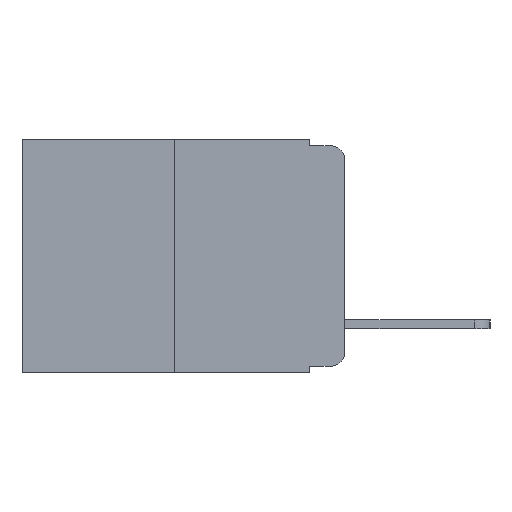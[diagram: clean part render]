
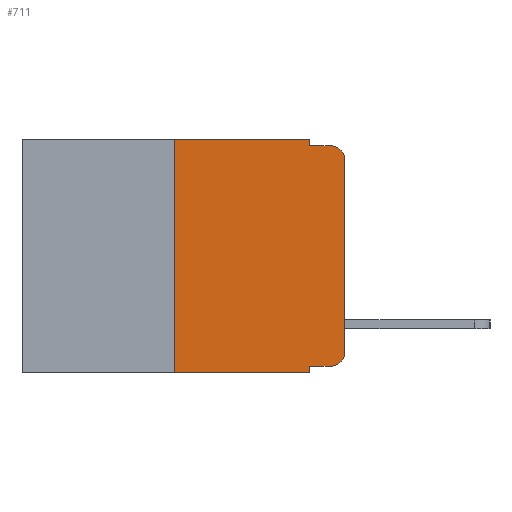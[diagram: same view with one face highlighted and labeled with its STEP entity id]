
A CAD part, left-side view. The second image highlights one B-rep face of the part: STEP entity #711.
In plain terms, the highlighted planar face has unit normal (-1, 0, 0).
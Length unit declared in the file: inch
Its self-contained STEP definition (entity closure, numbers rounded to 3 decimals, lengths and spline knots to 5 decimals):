
#6 = EDGE_CURVE ( 'NONE', #1286, #346, #4742, .T. ) ;
#98 = ORIENTED_EDGE ( 'NONE', *, *, #12733, .F. ) ;
#346 = VERTEX_POINT ( 'NONE', #18806 ) ;
#382 = DIRECTION ( 'NONE',  ( 0., 0., -1. ) ) ;
#711 = ADVANCED_FACE ( 'NONE', ( #3236 ), #2414, .F. ) ;
#789 = CARTESIAN_POINT ( 'NONE',  ( 0., 0.25, -0.343 ) ) ;
#946 = ORIENTED_EDGE ( 'NONE', *, *, #2792, .F. ) ;
#1286 = VERTEX_POINT ( 'NONE', #16000 ) ;
#1476 = DIRECTION ( 'NONE',  ( 0., -1., 0. ) ) ;
#1583 = EDGE_CURVE ( 'NONE', #17958, #12314, #21083, .T. ) ;
#1644 = CARTESIAN_POINT ( 'NONE',  ( 0., 0.051, -0.333 ) ) ;
#2068 = VECTOR ( 'NONE', #4440, 39.37008 ) ;
#2414 = PLANE ( 'NONE',  #10949 ) ;
#2440 = VERTEX_POINT ( 'NONE', #1644 ) ;
#2462 = VERTEX_POINT ( 'NONE', #10036 ) ;
#2792 = EDGE_CURVE ( 'NONE', #346, #12314, #10688, .T. ) ;
#3004 = CARTESIAN_POINT ( 'NONE',  ( 0., 0.02, -0.333 ) ) ;
#3225 = DIRECTION ( 'NONE',  ( 0., -1., 0. ) ) ;
#3236 = FACE_OUTER_BOUND ( 'NONE', #13621, .T. ) ;
#3529 = CARTESIAN_POINT ( 'NONE',  ( 0., 0.473, 0. ) ) ;
#3728 = ORIENTED_EDGE ( 'NONE', *, *, #13733, .F. ) ;
#4112 = CARTESIAN_POINT ( 'NONE',  ( 0., 0., -0.313 ) ) ;
#4440 = DIRECTION ( 'NONE',  ( 0., -1., 0. ) ) ;
#4742 = LINE ( 'NONE', #11547, #13829 ) ;
#5245 = LINE ( 'NONE', #5909, #13782 ) ;
#5909 = CARTESIAN_POINT ( 'NONE',  ( 0., 0.051, 0. ) ) ;
#6006 = LINE ( 'NONE', #8150, #10530 ) ;
#6038 = CARTESIAN_POINT ( 'NONE',  ( 0., 0.02, -0.01 ) ) ;
#6228 = LINE ( 'NONE', #16897, #13696 ) ;
#6269 = EDGE_CURVE ( 'NONE', #17419, #17958, #6540, .T. ) ;
#6456 = ORIENTED_EDGE ( 'NONE', *, *, #19779, .T. ) ;
#6540 = LINE ( 'NONE', #9797, #19561 ) ;
#7329 = LINE ( 'NONE', #13492, #20318 ) ;
#8150 = CARTESIAN_POINT ( 'NONE',  ( 0., 0.25, 0. ) ) ;
#9089 = CARTESIAN_POINT ( 'NONE',  ( 0., 0.473, 0. ) ) ;
#9797 = CARTESIAN_POINT ( 'NONE',  ( 0., 0., 0. ) ) ;
#10036 = CARTESIAN_POINT ( 'NONE',  ( 0., 0.051, -0.343 ) ) ;
#10133 = EDGE_CURVE ( 'NONE', #2440, #18264, #7329, .T. ) ;
#10244 = CARTESIAN_POINT ( 'NONE',  ( 0., 0.02, -0.313 ) ) ;
#10254 = CARTESIAN_POINT ( 'NONE',  ( 0., 0.25, 0. ) ) ;
#10530 = VECTOR ( 'NONE', #20041, 39.37008 ) ;
#10688 = LINE ( 'NONE', #14666, #2068 ) ;
#10728 = VERTEX_POINT ( 'NONE', #10254 ) ;
#10826 = AXIS2_PLACEMENT_3D ( 'NONE', #12504, #13002, #12960 ) ;
#10949 = AXIS2_PLACEMENT_3D ( 'NONE', #3529, #21132, #13618 ) ;
#11547 = CARTESIAN_POINT ( 'NONE',  ( 0., 0.051, 0. ) ) ;
#11979 = DIRECTION ( 'NONE',  ( 0., 0., -1. ) ) ;
#12314 = VERTEX_POINT ( 'NONE', #6038 ) ;
#12504 = CARTESIAN_POINT ( 'NONE',  ( 0., 0.02, -0.03 ) ) ;
#12733 = EDGE_CURVE ( 'NONE', #21360, #10728, #6006, .T. ) ;
#12960 = DIRECTION ( 'NONE',  ( 0., 0., -1. ) ) ;
#13002 = DIRECTION ( 'NONE',  ( -1., 0., 0. ) ) ;
#13492 = CARTESIAN_POINT ( 'NONE',  ( 0., 0.051, -0.333 ) ) ;
#13618 = DIRECTION ( 'NONE',  ( 0., 0., -1. ) ) ;
#13621 = EDGE_LOOP ( 'NONE', ( #20764, #13632, #946, #15211, #3728, #98, #6456, #17050, #16271, #21315 ) ) ;
#13632 = ORIENTED_EDGE ( 'NONE', *, *, #1583, .T. ) ;
#13696 = VECTOR ( 'NONE', #1476, 39.37008 ) ;
#13733 = EDGE_CURVE ( 'NONE', #10728, #1286, #20079, .T. ) ;
#13782 = VECTOR ( 'NONE', #21196, 39.37008 ) ;
#13829 = VECTOR ( 'NONE', #382, 39.37008 ) ;
#14125 = CARTESIAN_POINT ( 'NONE',  ( 0., 0., -0.03 ) ) ;
#14666 = CARTESIAN_POINT ( 'NONE',  ( 0., 0.051, -0.01 ) ) ;
#15211 = ORIENTED_EDGE ( 'NONE', *, *, #6, .F. ) ;
#15540 = VECTOR ( 'NONE', #15815, 39.37008 ) ;
#15815 = DIRECTION ( 'NONE',  ( 0., -1., 0. ) ) ;
#16000 = CARTESIAN_POINT ( 'NONE',  ( 0., 0.051, 0. ) ) ;
#16015 = AXIS2_PLACEMENT_3D ( 'NONE', #10244, #22085, #11979 ) ;
#16271 = ORIENTED_EDGE ( 'NONE', *, *, #10133, .T. ) ;
#16897 = CARTESIAN_POINT ( 'NONE',  ( 0., 0.473, -0.343 ) ) ;
#17050 = ORIENTED_EDGE ( 'NONE', *, *, #18080, .F. ) ;
#17419 = VERTEX_POINT ( 'NONE', #4112 ) ;
#17958 = VERTEX_POINT ( 'NONE', #14125 ) ;
#18080 = EDGE_CURVE ( 'NONE', #2440, #2462, #5245, .T. ) ;
#18176 = CIRCLE ( 'NONE', #16015, 0.02 ) ;
#18264 = VERTEX_POINT ( 'NONE', #3004 ) ;
#18806 = CARTESIAN_POINT ( 'NONE',  ( 0., 0.051, -0.01 ) ) ;
#19561 = VECTOR ( 'NONE', #21629, 39.37008 ) ;
#19779 = EDGE_CURVE ( 'NONE', #21360, #2462, #6228, .T. ) ;
#19799 = EDGE_CURVE ( 'NONE', #18264, #17419, #18176, .T. ) ;
#20041 = DIRECTION ( 'NONE',  ( 0., 0., 1. ) ) ;
#20079 = LINE ( 'NONE', #9089, #15540 ) ;
#20318 = VECTOR ( 'NONE', #3225, 39.37008 ) ;
#20764 = ORIENTED_EDGE ( 'NONE', *, *, #6269, .T. ) ;
#21083 = CIRCLE ( 'NONE', #10826, 0.02 ) ;
#21132 = DIRECTION ( 'NONE',  ( 1., 0., 0. ) ) ;
#21196 = DIRECTION ( 'NONE',  ( 0., 0., -1. ) ) ;
#21315 = ORIENTED_EDGE ( 'NONE', *, *, #19799, .T. ) ;
#21360 = VERTEX_POINT ( 'NONE', #789 ) ;
#21629 = DIRECTION ( 'NONE',  ( 0., 0., 1. ) ) ;
#22085 = DIRECTION ( 'NONE',  ( -1., 0., 0. ) ) ;
